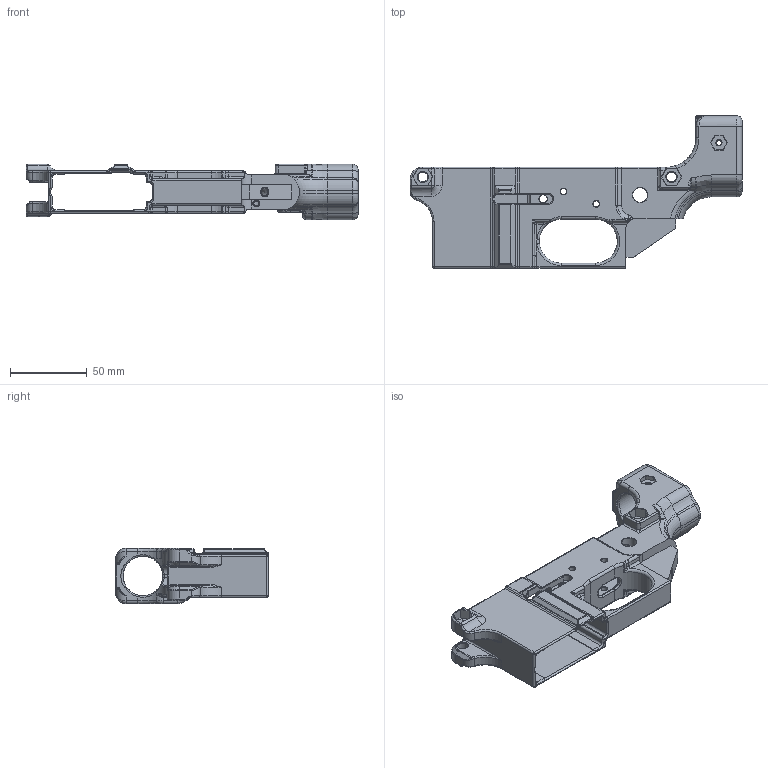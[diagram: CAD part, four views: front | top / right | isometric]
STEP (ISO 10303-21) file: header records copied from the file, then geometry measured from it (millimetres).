
FILE_DESCRIPTION(/* description */ (''),/* implementation_level */ '2;1');
FILE_NAME(/* name */ 'bbeacd76-b382-4321-9c8f-b886611aa2c8.stp',/* time_stamp */ '2019-04-30T20:49:01-04:00',/* author */ (''),/* organization */ (''),/* preprocessor_version */ 'ST-DEVELOPER v18',/* originating_system */ 'Autodesk Translation Framework v8.2.0.1029',/* authorisation */ '');
FILE_SCHEMA (('AUTOMOTIVE_DESIGN { 1 0 10303 214 3 1 1 }'));
Length unit declared in the file: millimetre
Products named in the file (1): FusionComponent
Bounding box: 216.15 x 99.32 x 36 mm (x, y, z)
Volume: 133784.8 mm3; surface area: 58310.2 mm2
Topology: 1 solids, 1 shells, 831 faces, 2054 edges, 1182 vertices
Faces by surface type: cylinder 252, bspline 200, plane 187, torus 123, cone 43, sphere 26
Full cylindrical faces by diameter (mm): 3 x2, 3.175 x1, 3.962 x5, 5.232 x1, 6.375 x4, 8.077 x1, 9.58 x2, 25.75 x1
Entity records: 31391 total; most frequent: CARTESIAN_POINT 12774, ORIENTED_EDGE 4038, DIRECTION 3728, EDGE_CURVE 2019, AXIS2_PLACEMENT_3D 1470, VERTEX_POINT 1182, EDGE_LOOP 859, FACE_OUTER_BOUND 829
